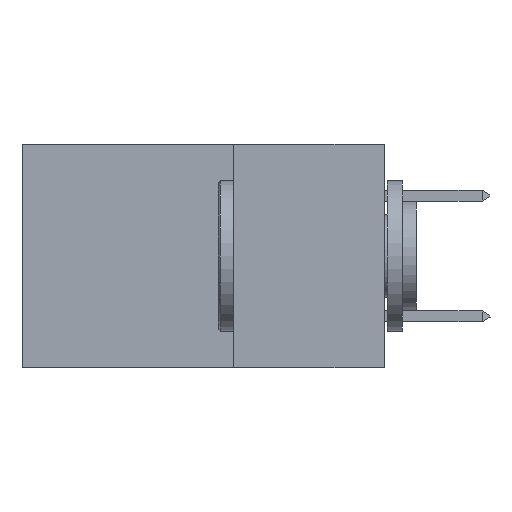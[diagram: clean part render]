
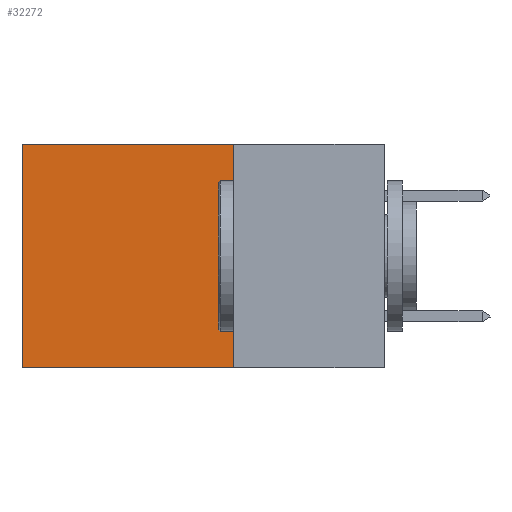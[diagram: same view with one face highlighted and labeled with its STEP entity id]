
A CAD part, left-side view. The second image highlights one B-rep face of the part: STEP entity #32272.
In plain terms, the highlighted planar face has unit normal (-1, 0, 0).
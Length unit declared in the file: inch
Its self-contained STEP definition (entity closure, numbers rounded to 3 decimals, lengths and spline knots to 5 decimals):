
#1393 = VECTOR ( 'NONE', #18795, 39.37008 ) ;
#1663 = VERTEX_POINT ( 'NONE', #27650 ) ;
#2076 = EDGE_LOOP ( 'NONE', ( #26211, #17622, #7832, #3407 ) ) ;
#3407 = ORIENTED_EDGE ( 'NONE', *, *, #13414, .T. ) ;
#3809 = LINE ( 'NONE', #10591, #12292 ) ;
#6862 = DIRECTION ( 'NONE',  ( 1., 0., 0. ) ) ;
#7832 = ORIENTED_EDGE ( 'NONE', *, *, #26965, .F. ) ;
#9020 = DIRECTION ( 'NONE',  ( 0., 1., 0. ) ) ;
#9308 = LINE ( 'NONE', #22126, #22754 ) ;
#10553 = VERTEX_POINT ( 'NONE', #10944 ) ;
#10591 = CARTESIAN_POINT ( 'NONE',  ( 0.2875, 0.6, 0. ) ) ;
#10944 = CARTESIAN_POINT ( 'NONE',  ( 0.2875, 0.6, -0.37 ) ) ;
#11268 = DIRECTION ( 'NONE',  ( 0., 0., -1. ) ) ;
#12096 = DIRECTION ( 'NONE',  ( 0., 0., -1. ) ) ;
#12292 = VECTOR ( 'NONE', #21038, 39.37008 ) ;
#13414 = EDGE_CURVE ( 'NONE', #1663, #19029, #9308, .T. ) ;
#15441 = EDGE_CURVE ( 'NONE', #19029, #10553, #3809, .T. ) ;
#17622 = ORIENTED_EDGE ( 'NONE', *, *, #20796, .F. ) ;
#17623 = LINE ( 'NONE', #31859, #1393 ) ;
#18795 = DIRECTION ( 'NONE',  ( 0., 1., 0. ) ) ;
#18960 = CARTESIAN_POINT ( 'NONE',  ( 0.2875, 0.25, 0. ) ) ;
#19029 = VERTEX_POINT ( 'NONE', #33189 ) ;
#19144 = VERTEX_POINT ( 'NONE', #23454 ) ;
#20605 = VECTOR ( 'NONE', #11268, 39.37008 ) ;
#20796 = EDGE_CURVE ( 'NONE', #19144, #10553, #17623, .T. ) ;
#21038 = DIRECTION ( 'NONE',  ( 0., 0., -1. ) ) ;
#22126 = CARTESIAN_POINT ( 'NONE',  ( 0.2875, 0.25, 0. ) ) ;
#22754 = VECTOR ( 'NONE', #9020, 39.37008 ) ;
#23454 = CARTESIAN_POINT ( 'NONE',  ( 0.2875, 0.25, -0.37 ) ) ;
#25140 = LINE ( 'NONE', #18960, #20605 ) ;
#26211 = ORIENTED_EDGE ( 'NONE', *, *, #15441, .T. ) ;
#26965 = EDGE_CURVE ( 'NONE', #1663, #19144, #25140, .T. ) ;
#27650 = CARTESIAN_POINT ( 'NONE',  ( 0.2875, 0.25, 0. ) ) ;
#27701 = PLANE ( 'NONE',  #28976 ) ;
#28976 = AXIS2_PLACEMENT_3D ( 'NONE', #32637, #6862, #12096 ) ;
#31381 = FACE_OUTER_BOUND ( 'NONE', #2076, .T. ) ;
#31859 = CARTESIAN_POINT ( 'NONE',  ( 0.2875, 0.25, -0.37 ) ) ;
#32272 = ADVANCED_FACE ( 'NONE', ( #31381 ), #27701, .F. ) ;
#32637 = CARTESIAN_POINT ( 'NONE',  ( 0.2875, 0.25, 0. ) ) ;
#33189 = CARTESIAN_POINT ( 'NONE',  ( 0.2875, 0.6, 0. ) ) ;
